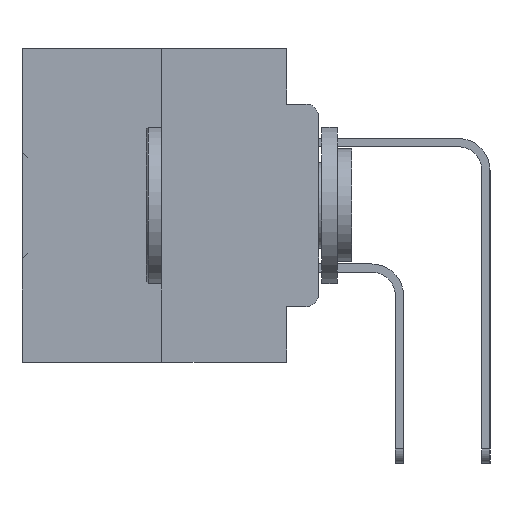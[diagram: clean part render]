
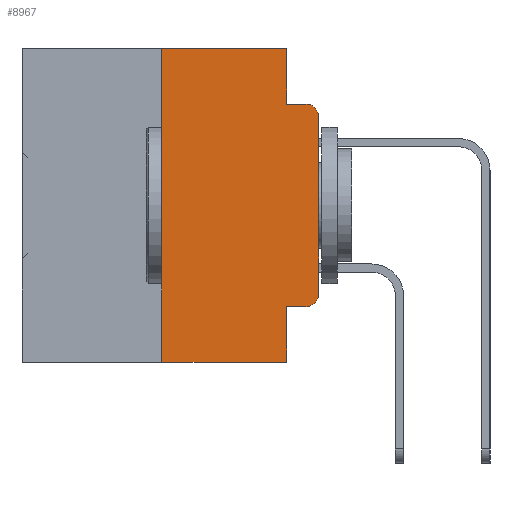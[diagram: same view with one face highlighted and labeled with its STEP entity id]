
A CAD part, left-side view. The second image highlights one B-rep face of the part: STEP entity #8967.
In plain terms, the highlighted planar face has unit normal (-1, 0, 0).
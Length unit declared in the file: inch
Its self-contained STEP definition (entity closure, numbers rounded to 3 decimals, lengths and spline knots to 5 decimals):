
#353 = ORIENTED_EDGE ( 'NONE', *, *, #5515, .T. ) ;
#667 = AXIS2_PLACEMENT_3D ( 'NONE', #28830, #23078, #5447 ) ;
#803 = CARTESIAN_POINT ( 'NONE',  ( 0., 0.25, 0. ) ) ;
#932 = CARTESIAN_POINT ( 'NONE',  ( 0., 0.473, -0.5 ) ) ;
#1298 = ORIENTED_EDGE ( 'NONE', *, *, #33725, .F. ) ;
#1716 = ORIENTED_EDGE ( 'NONE', *, *, #17241, .T. ) ;
#1825 = DIRECTION ( 'NONE',  ( 0., 0., 1. ) ) ;
#2099 = CARTESIAN_POINT ( 'NONE',  ( 0., 0., -0.1085 ) ) ;
#2105 = LINE ( 'NONE', #932, #16784 ) ;
#2164 = LINE ( 'NONE', #18698, #3060 ) ;
#2175 = VECTOR ( 'NONE', #13414, 39.37008 ) ;
#3060 = VECTOR ( 'NONE', #9928, 39.37008 ) ;
#3360 = CARTESIAN_POINT ( 'NONE',  ( 0., 0.051, -0.0885 ) ) ;
#3532 = CARTESIAN_POINT ( 'NONE',  ( 0., 0.02, -0.3915 ) ) ;
#3726 = DIRECTION ( 'NONE',  ( 0., 0., -1. ) ) ;
#3871 = DIRECTION ( 'NONE',  ( 0., -1., 0. ) ) ;
#5447 = DIRECTION ( 'NONE',  ( 0., 0., -1. ) ) ;
#5515 = EDGE_CURVE ( 'NONE', #8921, #23136, #25609, .T. ) ;
#5525 = EDGE_CURVE ( 'NONE', #22185, #35980, #2164, .T. ) ;
#5661 = CARTESIAN_POINT ( 'NONE',  ( 0., 0.02, -0.0885 ) ) ;
#6493 = DIRECTION ( 'NONE',  ( 0., 0., -1. ) ) ;
#6885 = FACE_OUTER_BOUND ( 'NONE', #23328, .T. ) ;
#7018 = DIRECTION ( 'NONE',  ( -1., 0., 0. ) ) ;
#7753 = VERTEX_POINT ( 'NONE', #35090 ) ;
#7775 = ORIENTED_EDGE ( 'NONE', *, *, #28525, .T. ) ;
#8440 = VERTEX_POINT ( 'NONE', #14393 ) ;
#8921 = VERTEX_POINT ( 'NONE', #2099 ) ;
#8967 = ADVANCED_FACE ( 'NONE', ( #6885 ), #20080, .F. ) ;
#9217 = CARTESIAN_POINT ( 'NONE',  ( 0., 0., -0.3915 ) ) ;
#9507 = ORIENTED_EDGE ( 'NONE', *, *, #19398, .F. ) ;
#9928 = DIRECTION ( 'NONE',  ( 0., 0., -1. ) ) ;
#10020 = ORIENTED_EDGE ( 'NONE', *, *, #35053, .T. ) ;
#10154 = VECTOR ( 'NONE', #1825, 39.37008 ) ;
#11149 = VERTEX_POINT ( 'NONE', #803 ) ;
#12279 = VECTOR ( 'NONE', #16166, 39.37008 ) ;
#12456 = CARTESIAN_POINT ( 'NONE',  ( 0., 0.051, -0.4115 ) ) ;
#12643 = LINE ( 'NONE', #30743, #27457 ) ;
#13414 = DIRECTION ( 'NONE',  ( 0., -1., 0. ) ) ;
#14393 = CARTESIAN_POINT ( 'NONE',  ( 0., 0.02, -0.4115 ) ) ;
#14567 = ORIENTED_EDGE ( 'NONE', *, *, #20852, .T. ) ;
#15319 = AXIS2_PLACEMENT_3D ( 'NONE', #3532, #24112, #6493 ) ;
#16166 = DIRECTION ( 'NONE',  ( 0., -1., 0. ) ) ;
#16784 = VECTOR ( 'NONE', #3871, 39.37008 ) ;
#16816 = VERTEX_POINT ( 'NONE', #17361 ) ;
#17241 = EDGE_CURVE ( 'NONE', #17495, #8921, #33638, .T. ) ;
#17361 = CARTESIAN_POINT ( 'NONE',  ( 0., 0.25, -0.5 ) ) ;
#17495 = VERTEX_POINT ( 'NONE', #9217 ) ;
#18698 = CARTESIAN_POINT ( 'NONE',  ( 0., 0.051, 0. ) ) ;
#19093 = CARTESIAN_POINT ( 'NONE',  ( 0., 0.051, -0.4115 ) ) ;
#19281 = LINE ( 'NONE', #27905, #12279 ) ;
#19306 = AXIS2_PLACEMENT_3D ( 'NONE', #24633, #7018, #27587 ) ;
#19398 = EDGE_CURVE ( 'NONE', #7753, #23851, #30271, .T. ) ;
#19935 = CARTESIAN_POINT ( 'NONE',  ( 0., 0.051, -0.5 ) ) ;
#20080 = PLANE ( 'NONE',  #667 ) ;
#20852 = EDGE_CURVE ( 'NONE', #16816, #35980, #2105, .T. ) ;
#22185 = VERTEX_POINT ( 'NONE', #19093 ) ;
#22972 = ORIENTED_EDGE ( 'NONE', *, *, #5525, .F. ) ;
#23078 = DIRECTION ( 'NONE',  ( 1., 0., 0. ) ) ;
#23136 = VERTEX_POINT ( 'NONE', #5661 ) ;
#23328 = EDGE_LOOP ( 'NONE', ( #1716, #353, #32531, #9507, #37504, #1298, #14567, #22972, #10020, #7775 ) ) ;
#23851 = VERTEX_POINT ( 'NONE', #3360 ) ;
#24112 = DIRECTION ( 'NONE',  ( -1., 0., 0. ) ) ;
#24247 = CIRCLE ( 'NONE', #15319, 0.02 ) ;
#24309 = CARTESIAN_POINT ( 'NONE',  ( 0., 0.051, 0. ) ) ;
#24633 = CARTESIAN_POINT ( 'NONE',  ( 0., 0.02, -0.1085 ) ) ;
#25609 = CIRCLE ( 'NONE', #19306, 0.02 ) ;
#25622 = LINE ( 'NONE', #34039, #2175 ) ;
#27457 = VECTOR ( 'NONE', #33669, 39.37008 ) ;
#27587 = DIRECTION ( 'NONE',  ( 0., 0., -1. ) ) ;
#27905 = CARTESIAN_POINT ( 'NONE',  ( 0., 0.473, 0. ) ) ;
#28525 = EDGE_CURVE ( 'NONE', #8440, #17495, #24247, .T. ) ;
#28830 = CARTESIAN_POINT ( 'NONE',  ( 0., 0.473, 0. ) ) ;
#29565 = VECTOR ( 'NONE', #30168, 39.37008 ) ;
#30168 = DIRECTION ( 'NONE',  ( 0., -1., 0. ) ) ;
#30271 = LINE ( 'NONE', #24309, #31163 ) ;
#30743 = CARTESIAN_POINT ( 'NONE',  ( 0., 0.25, 0. ) ) ;
#31163 = VECTOR ( 'NONE', #3726, 39.37008 ) ;
#31969 = EDGE_CURVE ( 'NONE', #11149, #7753, #19281, .T. ) ;
#32531 = ORIENTED_EDGE ( 'NONE', *, *, #33821, .F. ) ;
#33638 = LINE ( 'NONE', #36910, #10154 ) ;
#33669 = DIRECTION ( 'NONE',  ( 0., 0., 1. ) ) ;
#33725 = EDGE_CURVE ( 'NONE', #16816, #11149, #12643, .T. ) ;
#33821 = EDGE_CURVE ( 'NONE', #23851, #23136, #25622, .T. ) ;
#34039 = CARTESIAN_POINT ( 'NONE',  ( 0., 0.051, -0.0885 ) ) ;
#35053 = EDGE_CURVE ( 'NONE', #22185, #8440, #37264, .T. ) ;
#35090 = CARTESIAN_POINT ( 'NONE',  ( 0., 0.051, 0. ) ) ;
#35980 = VERTEX_POINT ( 'NONE', #19935 ) ;
#36910 = CARTESIAN_POINT ( 'NONE',  ( 0., 0., 0. ) ) ;
#37264 = LINE ( 'NONE', #12456, #29565 ) ;
#37504 = ORIENTED_EDGE ( 'NONE', *, *, #31969, .F. ) ;
